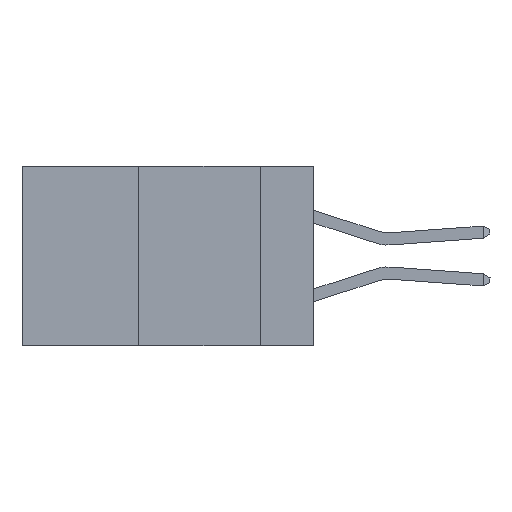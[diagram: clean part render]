
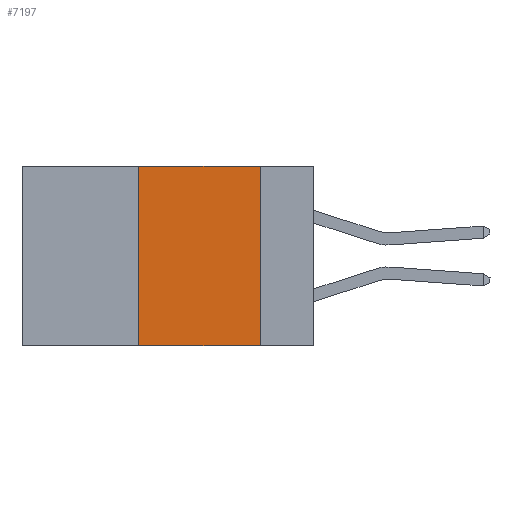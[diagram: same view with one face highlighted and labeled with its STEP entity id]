
A CAD part, left-side view. The second image highlights one B-rep face of the part: STEP entity #7197.
In plain terms, the highlighted planar face has unit normal (-1, 0, 0).
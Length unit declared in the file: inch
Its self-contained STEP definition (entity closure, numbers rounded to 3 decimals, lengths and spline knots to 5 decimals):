
#167 = VECTOR ( 'NONE', #4338, 39.37008 ) ;
#737 = FACE_OUTER_BOUND ( 'NONE', #2153, .T. ) ;
#2004 = EDGE_CURVE ( 'NONE', #8369, #28600, #20503, .T. ) ;
#2153 = EDGE_LOOP ( 'NONE', ( #22596, #8486, #22664, #11614 ) ) ;
#2551 = VERTEX_POINT ( 'NONE', #6586 ) ;
#3120 = CARTESIAN_POINT ( 'NONE',  ( 0., 0.11, -0.37 ) ) ;
#3589 = LINE ( 'NONE', #26973, #3829 ) ;
#3829 = VECTOR ( 'NONE', #20496, 39.37008 ) ;
#4030 = CARTESIAN_POINT ( 'NONE',  ( 0., 0.11, 0. ) ) ;
#4338 = DIRECTION ( 'NONE',  ( 0., 0., -1. ) ) ;
#5159 = AXIS2_PLACEMENT_3D ( 'NONE', #16407, #19476, #13168 ) ;
#6586 = CARTESIAN_POINT ( 'NONE',  ( 0., 0.11, 0. ) ) ;
#6654 = LINE ( 'NONE', #11264, #12156 ) ;
#7197 = ADVANCED_FACE ( 'NONE', ( #737 ), #23645, .F. ) ;
#8369 = VERTEX_POINT ( 'NONE', #9814 ) ;
#8486 = ORIENTED_EDGE ( 'NONE', *, *, #21598, .F. ) ;
#8833 = CARTESIAN_POINT ( 'NONE',  ( 0., 0.36, 0. ) ) ;
#9599 = EDGE_CURVE ( 'NONE', #2551, #17173, #15560, .T. ) ;
#9814 = CARTESIAN_POINT ( 'NONE',  ( 0., 0.36, -0.37 ) ) ;
#11264 = CARTESIAN_POINT ( 'NONE',  ( 0., 0.6, -0.37 ) ) ;
#11550 = VECTOR ( 'NONE', #25264, 39.37008 ) ;
#11614 = ORIENTED_EDGE ( 'NONE', *, *, #21772, .T. ) ;
#12156 = VECTOR ( 'NONE', #25256, 39.37008 ) ;
#13168 = DIRECTION ( 'NONE',  ( 0., 0., -1. ) ) ;
#14526 = CARTESIAN_POINT ( 'NONE',  ( 0., 0.36, 0. ) ) ;
#15560 = LINE ( 'NONE', #4030, #167 ) ;
#16407 = CARTESIAN_POINT ( 'NONE',  ( 0., 0.6, 0. ) ) ;
#17173 = VERTEX_POINT ( 'NONE', #3120 ) ;
#19476 = DIRECTION ( 'NONE',  ( 1., 0., 0. ) ) ;
#20496 = DIRECTION ( 'NONE',  ( 0., -1., 0. ) ) ;
#20503 = LINE ( 'NONE', #8833, #11550 ) ;
#21598 = EDGE_CURVE ( 'NONE', #28600, #2551, #3589, .T. ) ;
#21772 = EDGE_CURVE ( 'NONE', #8369, #17173, #6654, .T. ) ;
#22596 = ORIENTED_EDGE ( 'NONE', *, *, #9599, .F. ) ;
#22664 = ORIENTED_EDGE ( 'NONE', *, *, #2004, .F. ) ;
#23645 = PLANE ( 'NONE',  #5159 ) ;
#25256 = DIRECTION ( 'NONE',  ( 0., -1., 0. ) ) ;
#25264 = DIRECTION ( 'NONE',  ( 0., 0., 1. ) ) ;
#26973 = CARTESIAN_POINT ( 'NONE',  ( 0., 0.6, 0. ) ) ;
#28600 = VERTEX_POINT ( 'NONE', #14526 ) ;
